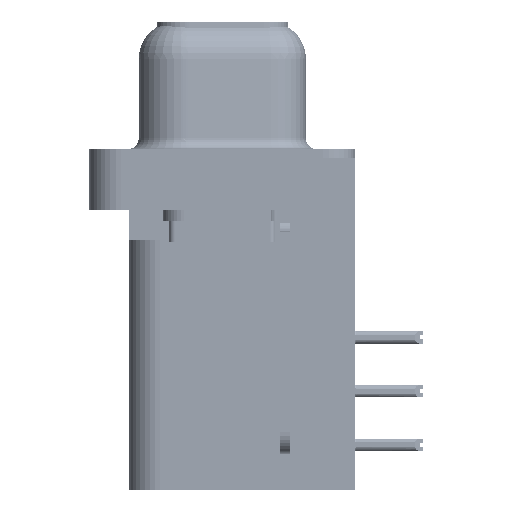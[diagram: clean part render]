
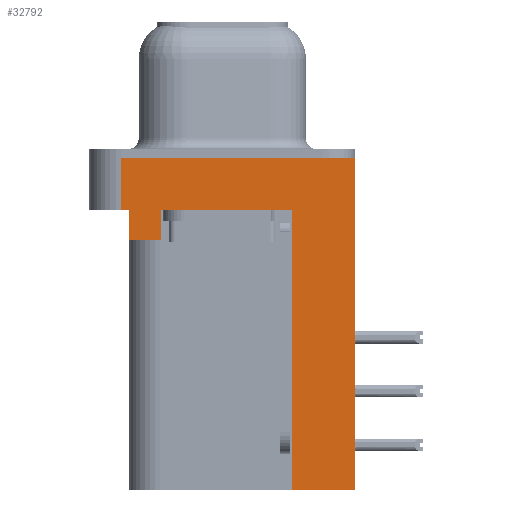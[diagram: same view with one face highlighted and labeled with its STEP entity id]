
A CAD part, left-side view. The second image highlights one B-rep face of the part: STEP entity #32792.
In plain terms, the highlighted planar face has unit normal (-1, 0, 0).
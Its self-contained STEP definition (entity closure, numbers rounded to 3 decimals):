
#201 = EDGE_CURVE ( 'NONE', #39028, #4519, #4731, .T. ) ;
#734 = DIRECTION ( 'NONE',  ( 0., -1., 0. ) ) ;
#1146 = CARTESIAN_POINT ( 'NONE',  ( -3., -6.275, 0. ) ) ;
#1438 = DIRECTION ( 'NONE',  ( 0., 1., 0. ) ) ;
#1831 = VECTOR ( 'NONE', #1438, 1000. ) ;
#1887 = ORIENTED_EDGE ( 'NONE', *, *, #9618, .T. ) ;
#2276 = LINE ( 'NONE', #35607, #1831 ) ;
#2505 = VECTOR ( 'NONE', #4586, 1000. ) ;
#2545 = LINE ( 'NONE', #11216, #2505 ) ;
#3317 = EDGE_CURVE ( 'NONE', #18522, #7231, #30228, .T. ) ;
#3611 = CARTESIAN_POINT ( 'NONE',  ( -3., 2.895, -2.5 ) ) ;
#3903 = CARTESIAN_POINT ( 'NONE',  ( -3., -6.275, -2.5 ) ) ;
#4302 = VECTOR ( 'NONE', #12791, 1000. ) ;
#4519 = VERTEX_POINT ( 'NONE', #25299 ) ;
#4586 = DIRECTION ( 'NONE',  ( 0., 0., 1. ) ) ;
#4633 = VECTOR ( 'NONE', #34059, 1000. ) ;
#4640 = LINE ( 'NONE', #6723, #4633 ) ;
#4731 = LINE ( 'NONE', #10867, #4302 ) ;
#5612 = ORIENTED_EDGE ( 'NONE', *, *, #201, .F. ) ;
#5991 = CARTESIAN_POINT ( 'NONE',  ( -3., 4.425, -3.9 ) ) ;
#6185 = CARTESIAN_POINT ( 'NONE',  ( -3., -3.295, -15.7 ) ) ;
#6273 = ORIENTED_EDGE ( 'NONE', *, *, #8110, .T. ) ;
#6723 = CARTESIAN_POINT ( 'NONE',  ( -3., 4.775, -2.5 ) ) ;
#7231 = VERTEX_POINT ( 'NONE', #27228 ) ;
#7448 = CARTESIAN_POINT ( 'NONE',  ( -3., -3.295, -2.5 ) ) ;
#7855 = EDGE_CURVE ( 'NONE', #33187, #18522, #4640, .T. ) ;
#8110 = EDGE_CURVE ( 'NONE', #29113, #7231, #2545, .T. ) ;
#8232 = CARTESIAN_POINT ( 'NONE',  ( -3., 2.895, -3.9 ) ) ;
#8423 = VERTEX_POINT ( 'NONE', #3611 ) ;
#8540 = VECTOR ( 'NONE', #734, 1000. ) ;
#9481 = DIRECTION ( 'NONE',  ( 0., 1., 0. ) ) ;
#9618 = EDGE_CURVE ( 'NONE', #15756, #8423, #32770, .T. ) ;
#10563 = CARTESIAN_POINT ( 'NONE',  ( -3., 4.775, 0. ) ) ;
#10863 = DIRECTION ( 'NONE',  ( 0., 0., 1. ) ) ;
#10867 = CARTESIAN_POINT ( 'NONE',  ( -3., 4.425, -3.9 ) ) ;
#11215 = LINE ( 'NONE', #39387, #28289 ) ;
#11216 = CARTESIAN_POINT ( 'NONE',  ( -3., -6.275, -2.5 ) ) ;
#11665 = VERTEX_POINT ( 'NONE', #42528 ) ;
#12197 = EDGE_CURVE ( 'NONE', #15756, #39028, #2276, .T. ) ;
#12791 = DIRECTION ( 'NONE',  ( 0., 0., 1. ) ) ;
#12953 = ORIENTED_EDGE ( 'NONE', *, *, #3317, .F. ) ;
#13757 = CARTESIAN_POINT ( 'NONE',  ( -3., 2.895, -3.9 ) ) ;
#14624 = FACE_OUTER_BOUND ( 'NONE', #25540, .T. ) ;
#15358 = DIRECTION ( 'NONE',  ( 0., 0., 1. ) ) ;
#15756 = VERTEX_POINT ( 'NONE', #8232 ) ;
#16040 = VERTEX_POINT ( 'NONE', #7448 ) ;
#17214 = EDGE_CURVE ( 'NONE', #29113, #11665, #26909, .T. ) ;
#17562 = EDGE_CURVE ( 'NONE', #33187, #4519, #24877, .T. ) ;
#17875 = CARTESIAN_POINT ( 'NONE',  ( -3., -6.275, -2.5 ) ) ;
#18126 = CARTESIAN_POINT ( 'NONE',  ( -3., -6.275, -15.7 ) ) ;
#18522 = VERTEX_POINT ( 'NONE', #10563 ) ;
#22961 = CARTESIAN_POINT ( 'NONE',  ( -3., 4.775, -2.5 ) ) ;
#24375 = PLANE ( 'NONE',  #29913 ) ;
#24666 = VECTOR ( 'NONE', #25202, 1000. ) ;
#24877 = LINE ( 'NONE', #42454, #24666 ) ;
#25127 = DIRECTION ( 'NONE',  ( 0., -1., 0. ) ) ;
#25202 = DIRECTION ( 'NONE',  ( 0., -1., 0. ) ) ;
#25299 = CARTESIAN_POINT ( 'NONE',  ( -3., 4.425, -2.5 ) ) ;
#25356 = ORIENTED_EDGE ( 'NONE', *, *, #17214, .F. ) ;
#25540 = EDGE_LOOP ( 'NONE', ( #12953, #25603, #28863, #5612, #30490, #1887, #27465, #30419, #25356, #6273 ) ) ;
#25603 = ORIENTED_EDGE ( 'NONE', *, *, #7855, .F. ) ;
#26909 = LINE ( 'NONE', #6185, #26951 ) ;
#26951 = VECTOR ( 'NONE', #9481, 1000. ) ;
#27228 = CARTESIAN_POINT ( 'NONE',  ( -3., -6.275, 0. ) ) ;
#27465 = ORIENTED_EDGE ( 'NONE', *, *, #28509, .T. ) ;
#28289 = VECTOR ( 'NONE', #15358, 1000. ) ;
#28509 = EDGE_CURVE ( 'NONE', #8423, #16040, #35785, .T. ) ;
#28700 = EDGE_CURVE ( 'NONE', #11665, #16040, #11215, .T. ) ;
#28863 = ORIENTED_EDGE ( 'NONE', *, *, #17562, .T. ) ;
#29113 = VERTEX_POINT ( 'NONE', #18126 ) ;
#29913 = AXIS2_PLACEMENT_3D ( 'NONE', #3903, #31277, #10863 ) ;
#30178 = VECTOR ( 'NONE', #25127, 1000. ) ;
#30228 = LINE ( 'NONE', #1146, #30178 ) ;
#30419 = ORIENTED_EDGE ( 'NONE', *, *, #28700, .F. ) ;
#30490 = ORIENTED_EDGE ( 'NONE', *, *, #12197, .F. ) ;
#31277 = DIRECTION ( 'NONE',  ( -1., 0., 0. ) ) ;
#32441 = VECTOR ( 'NONE', #41228, 1000. ) ;
#32770 = LINE ( 'NONE', #13757, #32441 ) ;
#32792 = ADVANCED_FACE ( 'NONE', ( #14624 ), #24375, .T. ) ;
#33187 = VERTEX_POINT ( 'NONE', #22961 ) ;
#34059 = DIRECTION ( 'NONE',  ( 0., 0., 1. ) ) ;
#35607 = CARTESIAN_POINT ( 'NONE',  ( -3., 4.425, -3.9 ) ) ;
#35785 = LINE ( 'NONE', #17875, #8540 ) ;
#39028 = VERTEX_POINT ( 'NONE', #5991 ) ;
#39387 = CARTESIAN_POINT ( 'NONE',  ( -3., -3.295, -15.7 ) ) ;
#41228 = DIRECTION ( 'NONE',  ( 0., 0., 1. ) ) ;
#42454 = CARTESIAN_POINT ( 'NONE',  ( -3., -6.275, -2.5 ) ) ;
#42528 = CARTESIAN_POINT ( 'NONE',  ( -3., -3.295, -15.7 ) ) ;
